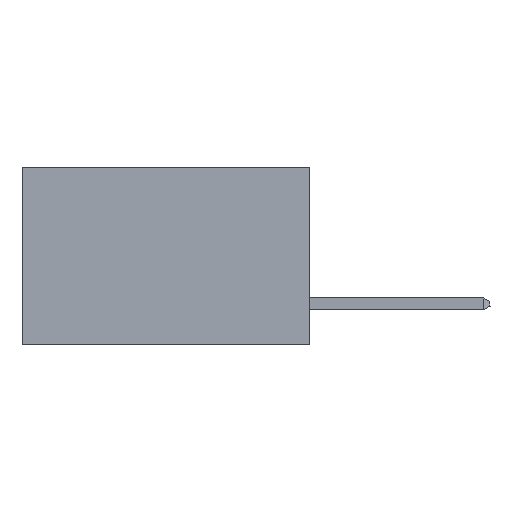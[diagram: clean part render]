
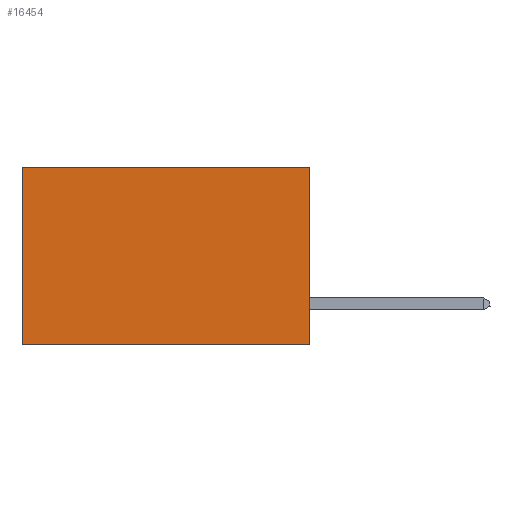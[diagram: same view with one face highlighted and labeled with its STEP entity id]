
A CAD part, left-side view. The second image highlights one B-rep face of the part: STEP entity #16454.
In plain terms, the highlighted planar face has unit normal (-1, 0, 0).
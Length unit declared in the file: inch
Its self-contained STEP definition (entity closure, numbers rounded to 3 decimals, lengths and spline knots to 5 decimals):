
#356 = ORIENTED_EDGE ( 'NONE', *, *, #33958, .T. ) ;
#586 = VERTEX_POINT ( 'NONE', #20113 ) ;
#692 = EDGE_CURVE ( 'NONE', #4041, #586, #11584, .T. ) ;
#3592 = CARTESIAN_POINT ( 'NONE',  ( 0.2875, 0., 0. ) ) ;
#4041 = VERTEX_POINT ( 'NONE', #3592 ) ;
#4228 = CARTESIAN_POINT ( 'NONE',  ( 0.2875, 0.6, -0.37 ) ) ;
#5132 = ORIENTED_EDGE ( 'NONE', *, *, #19555, .F. ) ;
#5849 = CARTESIAN_POINT ( 'NONE',  ( 0.2875, 0.6, 0. ) ) ;
#6400 = CARTESIAN_POINT ( 'NONE',  ( 0.2875, 0., 0. ) ) ;
#7311 = LINE ( 'NONE', #26936, #28114 ) ;
#9215 = DIRECTION ( 'NONE',  ( 0., 0., -1. ) ) ;
#9982 = CARTESIAN_POINT ( 'NONE',  ( 0.2875, 0.6, 0. ) ) ;
#11584 = LINE ( 'NONE', #32015, #25102 ) ;
#11644 = LINE ( 'NONE', #15853, #32985 ) ;
#12768 = DIRECTION ( 'NONE',  ( 0., 0., -1. ) ) ;
#14200 = VERTEX_POINT ( 'NONE', #5849 ) ;
#14908 = LINE ( 'NONE', #9982, #28300 ) ;
#15853 = CARTESIAN_POINT ( 'NONE',  ( 0.2875, 0., 0. ) ) ;
#16317 = DIRECTION ( 'NONE',  ( 0., 1., 0. ) ) ;
#16454 = ADVANCED_FACE ( 'NONE', ( #28420 ), #22798, .F. ) ;
#17815 = ORIENTED_EDGE ( 'NONE', *, *, #692, .F. ) ;
#18523 = DIRECTION ( 'NONE',  ( 0., 1., 0. ) ) ;
#19317 = VERTEX_POINT ( 'NONE', #4228 ) ;
#19555 = EDGE_CURVE ( 'NONE', #586, #19317, #7311, .T. ) ;
#20113 = CARTESIAN_POINT ( 'NONE',  ( 0.2875, 0., -0.37 ) ) ;
#21478 = AXIS2_PLACEMENT_3D ( 'NONE', #6400, #25441, #9215 ) ;
#21558 = DIRECTION ( 'NONE',  ( 0., 0., -1. ) ) ;
#22798 = PLANE ( 'NONE',  #21478 ) ;
#25102 = VECTOR ( 'NONE', #21558, 39.37008 ) ;
#25441 = DIRECTION ( 'NONE',  ( 1., 0., 0. ) ) ;
#25481 = EDGE_LOOP ( 'NONE', ( #356, #5132, #17815, #34071 ) ) ;
#26794 = EDGE_CURVE ( 'NONE', #4041, #14200, #11644, .T. ) ;
#26936 = CARTESIAN_POINT ( 'NONE',  ( 0.2875, 0., -0.37 ) ) ;
#28114 = VECTOR ( 'NONE', #16317, 39.37008 ) ;
#28300 = VECTOR ( 'NONE', #12768, 39.37008 ) ;
#28420 = FACE_OUTER_BOUND ( 'NONE', #25481, .T. ) ;
#32015 = CARTESIAN_POINT ( 'NONE',  ( 0.2875, 0., 0. ) ) ;
#32985 = VECTOR ( 'NONE', #18523, 39.37008 ) ;
#33958 = EDGE_CURVE ( 'NONE', #14200, #19317, #14908, .T. ) ;
#34071 = ORIENTED_EDGE ( 'NONE', *, *, #26794, .T. ) ;
